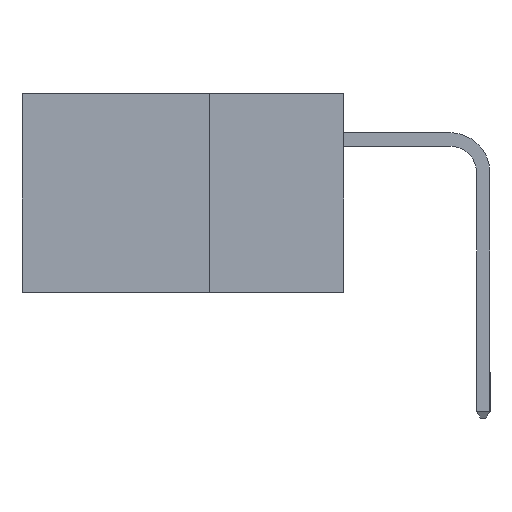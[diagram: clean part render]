
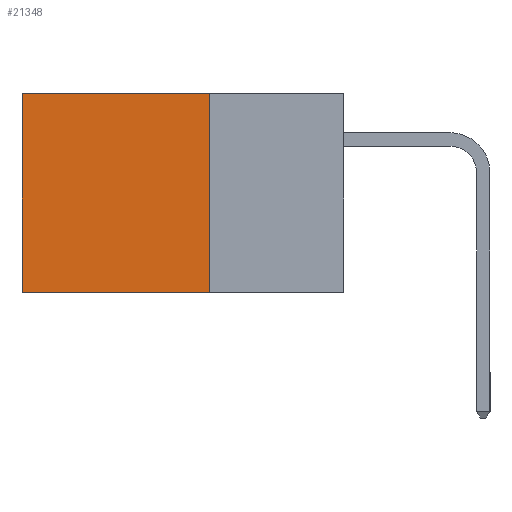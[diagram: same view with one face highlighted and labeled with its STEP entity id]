
A CAD part, left-side view. The second image highlights one B-rep face of the part: STEP entity #21348.
In plain terms, the highlighted planar face has unit normal (-1, 0, 0).
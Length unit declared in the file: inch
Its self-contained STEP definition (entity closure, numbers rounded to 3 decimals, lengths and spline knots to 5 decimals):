
#506 = DIRECTION ( 'NONE',  ( 0., 0., -1. ) ) ;
#860 = EDGE_CURVE ( 'NONE', #7644, #8486, #8726, .T. ) ;
#1121 = AXIS2_PLACEMENT_3D ( 'NONE', #2688, #22152, #506 ) ;
#1593 = CARTESIAN_POINT ( 'NONE',  ( 0.298, 0.6, -0.37 ) ) ;
#2149 = CARTESIAN_POINT ( 'NONE',  ( 0.298, 0.25, -0.37 ) ) ;
#2418 = LINE ( 'NONE', #14005, #11990 ) ;
#2507 = VECTOR ( 'NONE', #15824, 39.37008 ) ;
#2688 = CARTESIAN_POINT ( 'NONE',  ( 0.298, 0.25, 0. ) ) ;
#3256 = EDGE_CURVE ( 'NONE', #3707, #7644, #17027, .T. ) ;
#3276 = CARTESIAN_POINT ( 'NONE',  ( 0.298, 0.6, 0. ) ) ;
#3629 = CARTESIAN_POINT ( 'NONE',  ( 0.298, 0.25, 0. ) ) ;
#3707 = VERTEX_POINT ( 'NONE', #3629 ) ;
#7228 = DIRECTION ( 'NONE',  ( 0., 1., 0. ) ) ;
#7307 = FACE_OUTER_BOUND ( 'NONE', #23008, .T. ) ;
#7644 = VERTEX_POINT ( 'NONE', #15192 ) ;
#8486 = VERTEX_POINT ( 'NONE', #1593 ) ;
#8726 = LINE ( 'NONE', #3276, #2507 ) ;
#8889 = ORIENTED_EDGE ( 'NONE', *, *, #3256, .T. ) ;
#9252 = CARTESIAN_POINT ( 'NONE',  ( 0.298, 0.25, 0. ) ) ;
#10547 = VECTOR ( 'NONE', #7228, 39.37008 ) ;
#11990 = VECTOR ( 'NONE', #12114, 39.37008 ) ;
#12114 = DIRECTION ( 'NONE',  ( 0., 1., 0. ) ) ;
#13815 = VERTEX_POINT ( 'NONE', #2149 ) ;
#14005 = CARTESIAN_POINT ( 'NONE',  ( 0.298, 0.25, -0.37 ) ) ;
#14831 = LINE ( 'NONE', #20774, #18193 ) ;
#15092 = ORIENTED_EDGE ( 'NONE', *, *, #15758, .F. ) ;
#15192 = CARTESIAN_POINT ( 'NONE',  ( 0.298, 0.6, 0. ) ) ;
#15285 = DIRECTION ( 'NONE',  ( 0., 0., -1. ) ) ;
#15758 = EDGE_CURVE ( 'NONE', #13815, #8486, #2418, .T. ) ;
#15824 = DIRECTION ( 'NONE',  ( 0., 0., -1. ) ) ;
#17027 = LINE ( 'NONE', #9252, #10547 ) ;
#18193 = VECTOR ( 'NONE', #15285, 39.37008 ) ;
#19990 = ORIENTED_EDGE ( 'NONE', *, *, #22447, .F. ) ;
#20774 = CARTESIAN_POINT ( 'NONE',  ( 0.298, 0.25, 0. ) ) ;
#21348 = ADVANCED_FACE ( 'NONE', ( #7307 ), #22308, .F. ) ;
#22152 = DIRECTION ( 'NONE',  ( 1., 0., 0. ) ) ;
#22308 = PLANE ( 'NONE',  #1121 ) ;
#22447 = EDGE_CURVE ( 'NONE', #3707, #13815, #14831, .T. ) ;
#23008 = EDGE_LOOP ( 'NONE', ( #23299, #15092, #19990, #8889 ) ) ;
#23299 = ORIENTED_EDGE ( 'NONE', *, *, #860, .T. ) ;
